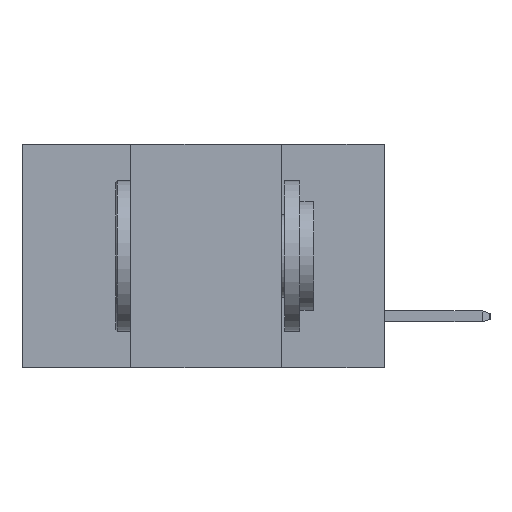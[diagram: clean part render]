
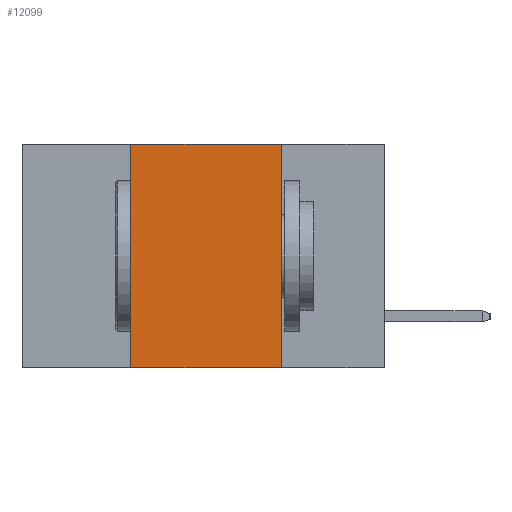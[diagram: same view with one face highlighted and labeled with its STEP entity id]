
A CAD part, left-side view. The second image highlights one B-rep face of the part: STEP entity #12099.
In plain terms, the highlighted planar face has unit normal (-1, 0, 0).
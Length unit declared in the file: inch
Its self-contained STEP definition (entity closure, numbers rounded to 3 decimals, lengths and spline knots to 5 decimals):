
#214 = VECTOR ( 'NONE', #2517, 39.37008 ) ;
#730 = LINE ( 'NONE', #869, #214 ) ;
#869 = CARTESIAN_POINT ( 'NONE',  ( 0., 0.6, 0. ) ) ;
#992 = PLANE ( 'NONE',  #17933 ) ;
#2175 = EDGE_CURVE ( 'NONE', #13014, #19730, #2553, .T. ) ;
#2410 = ORIENTED_EDGE ( 'NONE', *, *, #19636, .T. ) ;
#2517 = DIRECTION ( 'NONE',  ( 0., -1., 0. ) ) ;
#2553 = LINE ( 'NONE', #7184, #6274 ) ;
#2623 = DIRECTION ( 'NONE',  ( 1., 0., 0. ) ) ;
#3149 = CARTESIAN_POINT ( 'NONE',  ( 0., 0.17, -0.37 ) ) ;
#3435 = VECTOR ( 'NONE', #5200, 39.37008 ) ;
#3998 = VERTEX_POINT ( 'NONE', #14431 ) ;
#4574 = CARTESIAN_POINT ( 'NONE',  ( 0., 0.6, -0.37 ) ) ;
#4675 = ORIENTED_EDGE ( 'NONE', *, *, #5112, .F. ) ;
#5112 = EDGE_CURVE ( 'NONE', #3998, #19690, #16755, .T. ) ;
#5200 = DIRECTION ( 'NONE',  ( 0., 0., 1. ) ) ;
#5233 = DIRECTION ( 'NONE',  ( 0., 0., -1. ) ) ;
#5288 = CARTESIAN_POINT ( 'NONE',  ( 0., 0.42, -0.37 ) ) ;
#6142 = DIRECTION ( 'NONE',  ( 0., -1., 0. ) ) ;
#6274 = VECTOR ( 'NONE', #5233, 39.37008 ) ;
#7184 = CARTESIAN_POINT ( 'NONE',  ( 0., 0.17, -0.37 ) ) ;
#9174 = EDGE_LOOP ( 'NONE', ( #19231, #13982, #4675, #2410 ) ) ;
#11105 = FACE_OUTER_BOUND ( 'NONE', #9174, .T. ) ;
#12099 = ADVANCED_FACE ( 'NONE', ( #11105 ), #992, .F. ) ;
#12242 = CARTESIAN_POINT ( 'NONE',  ( 0., 0.6, 0. ) ) ;
#13014 = VERTEX_POINT ( 'NONE', #17954 ) ;
#13040 = LINE ( 'NONE', #4574, #17306 ) ;
#13289 = EDGE_CURVE ( 'NONE', #19690, #13014, #730, .T. ) ;
#13860 = DIRECTION ( 'NONE',  ( 0., 0., -1. ) ) ;
#13982 = ORIENTED_EDGE ( 'NONE', *, *, #13289, .F. ) ;
#14431 = CARTESIAN_POINT ( 'NONE',  ( 0., 0.42, -0.37 ) ) ;
#16755 = LINE ( 'NONE', #5288, #3435 ) ;
#17306 = VECTOR ( 'NONE', #6142, 39.37008 ) ;
#17933 = AXIS2_PLACEMENT_3D ( 'NONE', #12242, #2623, #13860 ) ;
#17954 = CARTESIAN_POINT ( 'NONE',  ( 0., 0.17, 0. ) ) ;
#19231 = ORIENTED_EDGE ( 'NONE', *, *, #2175, .F. ) ;
#19636 = EDGE_CURVE ( 'NONE', #3998, #19730, #13040, .T. ) ;
#19690 = VERTEX_POINT ( 'NONE', #20619 ) ;
#19730 = VERTEX_POINT ( 'NONE', #3149 ) ;
#20619 = CARTESIAN_POINT ( 'NONE',  ( 0., 0.42, 0. ) ) ;
